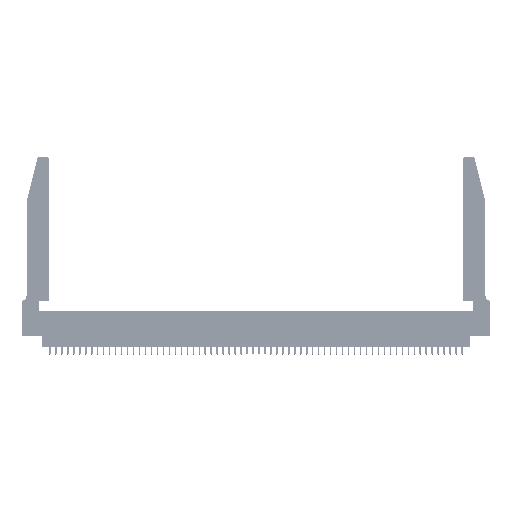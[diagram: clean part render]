
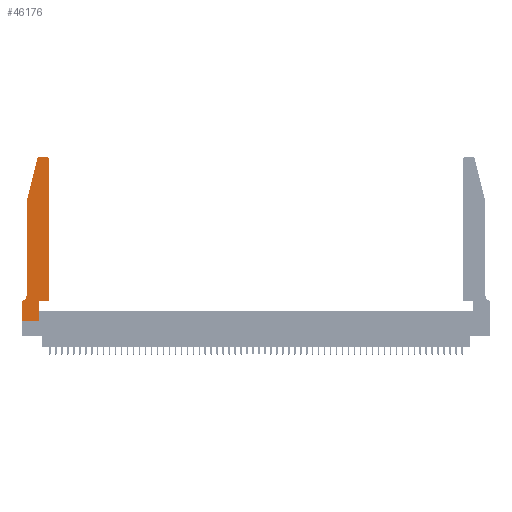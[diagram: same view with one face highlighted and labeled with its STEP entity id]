
A CAD part, top view. The second image highlights one B-rep face of the part: STEP entity #46176.
In plain terms, the highlighted planar face has unit normal (0, 0, 1).
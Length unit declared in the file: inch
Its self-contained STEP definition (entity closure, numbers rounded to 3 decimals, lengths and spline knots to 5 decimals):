
#69 = VERTEX_POINT ( 'NONE', #43856 ) ;
#551 = LINE ( 'NONE', #53755, #22271 ) ;
#1129 = CARTESIAN_POINT ( 'NONE',  ( 0.2865, 0.35, 0.37 ) ) ;
#1650 = CARTESIAN_POINT ( 'NONE',  ( 0.25487, 2.72718, 0.37 ) ) ;
#3069 = VECTOR ( 'NONE', #11286, 39.37008 ) ;
#4343 = DIRECTION ( 'NONE',  ( 1., 0., 0. ) ) ;
#6527 = EDGE_CURVE ( 'NONE', #28225, #9324, #9838, .T. ) ;
#7393 = CARTESIAN_POINT ( 'NONE',  ( 0.284, 2.72, 0.37 ) ) ;
#8029 = VECTOR ( 'NONE', #53822, 39.37008 ) ;
#8742 = AXIS2_PLACEMENT_3D ( 'NONE', #37647, #11782, #41978 ) ;
#9324 = VERTEX_POINT ( 'NONE', #21663 ) ;
#9714 = VERTEX_POINT ( 'NONE', #15374 ) ;
#9838 = LINE ( 'NONE', #43828, #41583 ) ;
#10128 = DIRECTION ( 'NONE',  ( -1., 0., 0. ) ) ;
#10458 = ORIENTED_EDGE ( 'NONE', *, *, #37450, .T. ) ;
#11286 = DIRECTION ( 'NONE',  ( 0., 1., 0. ) ) ;
#11715 = EDGE_CURVE ( 'NONE', #21719, #69, #27809, .T. ) ;
#11782 = DIRECTION ( 'NONE',  ( 0., 0., -1. ) ) ;
#11785 = DIRECTION ( 'NONE',  ( 1., 0., 0. ) ) ;
#11795 = EDGE_CURVE ( 'NONE', #30020, #21719, #35231, .T. ) ;
#12130 = EDGE_CURVE ( 'NONE', #40681, #26385, #17618, .T. ) ;
#12234 = VECTOR ( 'NONE', #10128, 39.37008 ) ;
#13634 = DIRECTION ( 'NONE',  ( -0.239, -0.971, 0. ) ) ;
#15374 = CARTESIAN_POINT ( 'NONE',  ( 0.2865, 0., 0.37 ) ) ;
#16240 = VERTEX_POINT ( 'NONE', #53653 ) ;
#17451 = LINE ( 'NONE', #37819, #51929 ) ;
#17618 = LINE ( 'NONE', #55280, #50735 ) ;
#17769 = CARTESIAN_POINT ( 'NONE',  ( 0.4205, 2.72, 0.37 ) ) ;
#19497 = ORIENTED_EDGE ( 'NONE', *, *, #12130, .T. ) ;
#19544 = ORIENTED_EDGE ( 'NONE', *, *, #45060, .T. ) ;
#19561 = LINE ( 'NONE', #40778, #8029 ) ;
#19784 = CARTESIAN_POINT ( 'NONE',  ( 0., 0.35, 0.37 ) ) ;
#20227 = CARTESIAN_POINT ( 'NONE',  ( 0.0755, 0.42, 0.37 ) ) ;
#20554 = EDGE_CURVE ( 'NONE', #69, #9714, #17451, .T. ) ;
#20899 = DIRECTION ( 'NONE',  ( 1., 0., 0. ) ) ;
#21592 = VECTOR ( 'NONE', #37900, 39.37008 ) ;
#21663 = CARTESIAN_POINT ( 'NONE',  ( 0.0755, 2., 0.37 ) ) ;
#21719 = VERTEX_POINT ( 'NONE', #36780 ) ;
#22271 = VECTOR ( 'NONE', #32220, 39.37008 ) ;
#22954 = CARTESIAN_POINT ( 'NONE',  ( 0.0055, 0.35, 0.37 ) ) ;
#23583 = ORIENTED_EDGE ( 'NONE', *, *, #39685, .T. ) ;
#24158 = DIRECTION ( 'NONE',  ( 1., 0., 0. ) ) ;
#24361 = VERTEX_POINT ( 'NONE', #46367 ) ;
#24798 = CARTESIAN_POINT ( 'NONE',  ( 0.4505, 0.35, 0.37 ) ) ;
#25664 = CIRCLE ( 'NONE', #41842, 0.03 ) ;
#26385 = VERTEX_POINT ( 'NONE', #24798 ) ;
#26992 = DIRECTION ( 'NONE',  ( 0., -1., 0. ) ) ;
#27809 = LINE ( 'NONE', #31319, #49431 ) ;
#28225 = VERTEX_POINT ( 'NONE', #1650 ) ;
#28765 = ORIENTED_EDGE ( 'NONE', *, *, #34250, .T. ) ;
#28793 = AXIS2_PLACEMENT_3D ( 'NONE', #17769, #30291, #4343 ) ;
#28843 = LINE ( 'NONE', #45865, #3069 ) ;
#29884 = CIRCLE ( 'NONE', #28793, 0.03 ) ;
#30020 = VERTEX_POINT ( 'NONE', #22954 ) ;
#30192 = ORIENTED_EDGE ( 'NONE', *, *, #6527, .T. ) ;
#30291 = DIRECTION ( 'NONE',  ( 0., 0., 1. ) ) ;
#31319 = CARTESIAN_POINT ( 'NONE',  ( 0., 0., 0.37 ) ) ;
#31371 = AXIS2_PLACEMENT_3D ( 'NONE', #19784, #50018, #24158 ) ;
#32220 = DIRECTION ( 'NONE',  ( -1., 0., 0. ) ) ;
#33043 = LINE ( 'NONE', #55139, #21592 ) ;
#34061 = EDGE_CURVE ( 'NONE', #16240, #24361, #551, .T. ) ;
#34250 = EDGE_CURVE ( 'NONE', #24361, #28225, #25664, .T. ) ;
#35231 = LINE ( 'NONE', #48887, #12234 ) ;
#35851 = FACE_OUTER_BOUND ( 'NONE', #46372, .T. ) ;
#36780 = CARTESIAN_POINT ( 'NONE',  ( 0., 0.35, 0.37 ) ) ;
#36973 = PLANE ( 'NONE',  #31371 ) ;
#37045 = ORIENTED_EDGE ( 'NONE', *, *, #52697, .T. ) ;
#37260 = EDGE_CURVE ( 'NONE', #9324, #47480, #19561, .T. ) ;
#37450 = EDGE_CURVE ( 'NONE', #9714, #40681, #33043, .T. ) ;
#37647 = CARTESIAN_POINT ( 'NONE',  ( 0.0055, 0.42, 0.37 ) ) ;
#37649 = DIRECTION ( 'NONE',  ( 0., 0., 1. ) ) ;
#37819 = CARTESIAN_POINT ( 'NONE',  ( 0., 0., 0.37 ) ) ;
#37900 = DIRECTION ( 'NONE',  ( 0., 1., 0. ) ) ;
#38426 = ORIENTED_EDGE ( 'NONE', *, *, #11795, .T. ) ;
#39685 = EDGE_CURVE ( 'NONE', #26385, #47669, #28843, .T. ) ;
#39705 = ORIENTED_EDGE ( 'NONE', *, *, #37260, .T. ) ;
#40369 = ORIENTED_EDGE ( 'NONE', *, *, #11715, .T. ) ;
#40681 = VERTEX_POINT ( 'NONE', #1129 ) ;
#40778 = CARTESIAN_POINT ( 'NONE',  ( 0.0755, 2., 0.37 ) ) ;
#41583 = VECTOR ( 'NONE', #13634, 39.37008 ) ;
#41842 = AXIS2_PLACEMENT_3D ( 'NONE', #7393, #37649, #11785 ) ;
#41978 = DIRECTION ( 'NONE',  ( -1., 0., 0. ) ) ;
#43828 = CARTESIAN_POINT ( 'NONE',  ( 0.0755, 2., 0.37 ) ) ;
#43856 = CARTESIAN_POINT ( 'NONE',  ( 0., 0., 0.37 ) ) ;
#44783 = CIRCLE ( 'NONE', #8742, 0.07 ) ;
#45060 = EDGE_CURVE ( 'NONE', #47669, #16240, #29884, .T. ) ;
#45865 = CARTESIAN_POINT ( 'NONE',  ( 0.4505, 0.35, 0.37 ) ) ;
#46176 = ADVANCED_FACE ( 'NONE', ( #35851 ), #36973, .T. ) ;
#46367 = CARTESIAN_POINT ( 'NONE',  ( 0.284, 2.75, 0.37 ) ) ;
#46372 = EDGE_LOOP ( 'NONE', ( #47849, #28765, #30192, #39705, #37045, #38426, #40369, #55284, #10458, #19497, #23583, #19544 ) ) ;
#47480 = VERTEX_POINT ( 'NONE', #20227 ) ;
#47669 = VERTEX_POINT ( 'NONE', #55947 ) ;
#47849 = ORIENTED_EDGE ( 'NONE', *, *, #34061, .T. ) ;
#48887 = CARTESIAN_POINT ( 'NONE',  ( 0.0755, 0.35, 0.37 ) ) ;
#49431 = VECTOR ( 'NONE', #26992, 39.37008 ) ;
#50018 = DIRECTION ( 'NONE',  ( 0., 0., 1. ) ) ;
#50735 = VECTOR ( 'NONE', #20899, 39.37008 ) ;
#51929 = VECTOR ( 'NONE', #55050, 39.37008 ) ;
#52697 = EDGE_CURVE ( 'NONE', #47480, #30020, #44783, .T. ) ;
#53653 = CARTESIAN_POINT ( 'NONE',  ( 0.4205, 2.75, 0.37 ) ) ;
#53755 = CARTESIAN_POINT ( 'NONE',  ( 0.2605, 2.75, 0.37 ) ) ;
#53822 = DIRECTION ( 'NONE',  ( 0., -1., 0. ) ) ;
#55050 = DIRECTION ( 'NONE',  ( 1., 0., 0. ) ) ;
#55139 = CARTESIAN_POINT ( 'NONE',  ( 0.2865, 0.35, 0.37 ) ) ;
#55280 = CARTESIAN_POINT ( 'NONE',  ( 0.4505, 0.35, 0.37 ) ) ;
#55284 = ORIENTED_EDGE ( 'NONE', *, *, #20554, .T. ) ;
#55947 = CARTESIAN_POINT ( 'NONE',  ( 0.4505, 2.72, 0.37 ) ) ;
